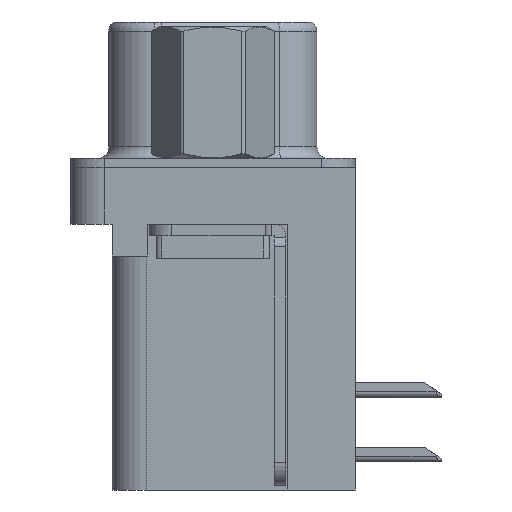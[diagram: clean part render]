
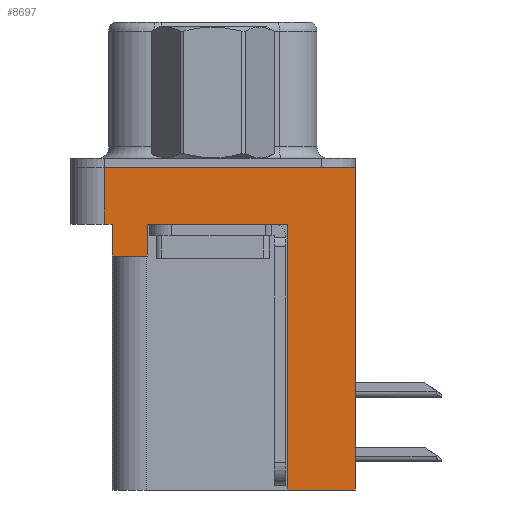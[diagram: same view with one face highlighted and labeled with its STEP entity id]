
A CAD part, left-side view. The second image highlights one B-rep face of the part: STEP entity #8697.
In plain terms, the highlighted planar face has unit normal (-1, 0, 0).
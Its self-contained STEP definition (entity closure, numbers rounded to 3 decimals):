
#73 = DIRECTION ( 'NONE',  ( 0., -1., 0. ) ) ;
#438 = VERTEX_POINT ( 'NONE', #10556 ) ;
#907 = EDGE_LOOP ( 'NONE', ( #11943, #14085, #15891, #15532, #23313, #14474, #13077, #6168, #18651, #9984 ) ) ;
#1224 = EDGE_CURVE ( 'NONE', #3925, #14186, #23632, .T. ) ;
#1886 = CARTESIAN_POINT ( 'NONE',  ( -2.935, -6.275, -2.5 ) ) ;
#2284 = CARTESIAN_POINT ( 'NONE',  ( -2.935, -6.275, 0. ) ) ;
#2301 = CARTESIAN_POINT ( 'NONE',  ( -2.935, -3.295, -14.2 ) ) ;
#2334 = PLANE ( 'NONE',  #7352 ) ;
#2431 = DIRECTION ( 'NONE',  ( 0., -1., 0. ) ) ;
#3066 = VERTEX_POINT ( 'NONE', #3614 ) ;
#3137 = EDGE_CURVE ( 'NONE', #3999, #21410, #13602, .T. ) ;
#3614 = CARTESIAN_POINT ( 'NONE',  ( -2.935, -3.295, -2.5 ) ) ;
#3846 = VECTOR ( 'NONE', #5718, 1000. ) ;
#3925 = VERTEX_POINT ( 'NONE', #4031 ) ;
#3999 = VERTEX_POINT ( 'NONE', #4621 ) ;
#4031 = CARTESIAN_POINT ( 'NONE',  ( -2.935, 4.775, -2.5 ) ) ;
#4054 = LINE ( 'NONE', #18849, #13269 ) ;
#4245 = CARTESIAN_POINT ( 'NONE',  ( -2.935, -6.275, -2.5 ) ) ;
#4557 = VECTOR ( 'NONE', #19603, 1000. ) ;
#4621 = CARTESIAN_POINT ( 'NONE',  ( -2.935, 2.895, -3.9 ) ) ;
#4792 = DIRECTION ( 'NONE',  ( 0., 0., 1. ) ) ;
#5610 = EDGE_CURVE ( 'NONE', #3999, #438, #23203, .T. ) ;
#5718 = DIRECTION ( 'NONE',  ( 0., 0., 1. ) ) ;
#5850 = DIRECTION ( 'NONE',  ( 0., 0., 1. ) ) ;
#6168 = ORIENTED_EDGE ( 'NONE', *, *, #19199, .F. ) ;
#7070 = CARTESIAN_POINT ( 'NONE',  ( -2.935, 2.895, -3.9 ) ) ;
#7352 = AXIS2_PLACEMENT_3D ( 'NONE', #17005, #11230, #18453 ) ;
#7708 = LINE ( 'NONE', #18665, #18121 ) ;
#7763 = VECTOR ( 'NONE', #10112, 1000. ) ;
#8419 = CARTESIAN_POINT ( 'NONE',  ( -2.935, -3.295, -14.2 ) ) ;
#8697 = ADVANCED_FACE ( 'NONE', ( #11104 ), #2334, .T. ) ;
#9215 = CARTESIAN_POINT ( 'NONE',  ( -2.935, 4.425, -3.9 ) ) ;
#9289 = VERTEX_POINT ( 'NONE', #12525 ) ;
#9972 = DIRECTION ( 'NONE',  ( 0., 1., 0. ) ) ;
#9984 = ORIENTED_EDGE ( 'NONE', *, *, #21409, .T. ) ;
#9987 = CARTESIAN_POINT ( 'NONE',  ( -2.935, -3.295, -14.2 ) ) ;
#10095 = VECTOR ( 'NONE', #9972, 1000. ) ;
#10112 = DIRECTION ( 'NONE',  ( 0., 1., 0. ) ) ;
#10114 = LINE ( 'NONE', #9987, #4557 ) ;
#10556 = CARTESIAN_POINT ( 'NONE',  ( -2.935, 2.895, -2.5 ) ) ;
#11104 = FACE_OUTER_BOUND ( 'NONE', #907, .T. ) ;
#11136 = LINE ( 'NONE', #1886, #3846 ) ;
#11230 = DIRECTION ( 'NONE',  ( -1., 0., 0. ) ) ;
#11920 = VECTOR ( 'NONE', #21591, 1000. ) ;
#11943 = ORIENTED_EDGE ( 'NONE', *, *, #23631, .F. ) ;
#12525 = CARTESIAN_POINT ( 'NONE',  ( -2.935, -6.275, -14.2 ) ) ;
#12873 = CARTESIAN_POINT ( 'NONE',  ( -2.935, 4.775, 0. ) ) ;
#13077 = ORIENTED_EDGE ( 'NONE', *, *, #17401, .T. ) ;
#13152 = CARTESIAN_POINT ( 'NONE',  ( -2.935, 4.425, -2.5 ) ) ;
#13269 = VECTOR ( 'NONE', #5850, 1000. ) ;
#13286 = DIRECTION ( 'NONE',  ( 0., -1., 0. ) ) ;
#13307 = EDGE_CURVE ( 'NONE', #21410, #14186, #4054, .T. ) ;
#13602 = LINE ( 'NONE', #19127, #10095 ) ;
#14085 = ORIENTED_EDGE ( 'NONE', *, *, #21740, .F. ) ;
#14131 = CARTESIAN_POINT ( 'NONE',  ( -2.935, 4.775, -2.5 ) ) ;
#14186 = VERTEX_POINT ( 'NONE', #13152 ) ;
#14474 = ORIENTED_EDGE ( 'NONE', *, *, #5610, .T. ) ;
#15532 = ORIENTED_EDGE ( 'NONE', *, *, #13307, .F. ) ;
#15571 = VERTEX_POINT ( 'NONE', #2284 ) ;
#15891 = ORIENTED_EDGE ( 'NONE', *, *, #1224, .T. ) ;
#16053 = VECTOR ( 'NONE', #13286, 1000. ) ;
#16526 = CARTESIAN_POINT ( 'NONE',  ( -2.935, -6.275, -2.5 ) ) ;
#16872 = LINE ( 'NONE', #4245, #16053 ) ;
#16911 = VECTOR ( 'NONE', #73, 1000. ) ;
#17005 = CARTESIAN_POINT ( 'NONE',  ( -2.935, -6.275, -2.5 ) ) ;
#17401 = EDGE_CURVE ( 'NONE', #438, #3066, #16872, .T. ) ;
#18121 = VECTOR ( 'NONE', #2431, 1000. ) ;
#18453 = DIRECTION ( 'NONE',  ( 0., 0., 1. ) ) ;
#18651 = ORIENTED_EDGE ( 'NONE', *, *, #23746, .F. ) ;
#18665 = CARTESIAN_POINT ( 'NONE',  ( -2.935, -6.275, 0. ) ) ;
#18849 = CARTESIAN_POINT ( 'NONE',  ( -2.935, 4.425, -3.9 ) ) ;
#19127 = CARTESIAN_POINT ( 'NONE',  ( -2.935, 4.425, -3.9 ) ) ;
#19199 = EDGE_CURVE ( 'NONE', #23633, #3066, #10114, .T. ) ;
#19603 = DIRECTION ( 'NONE',  ( 0., 0., 1. ) ) ;
#20715 = VECTOR ( 'NONE', #4792, 1000. ) ;
#20780 = VERTEX_POINT ( 'NONE', #12873 ) ;
#21409 = EDGE_CURVE ( 'NONE', #9289, #15571, #11136, .T. ) ;
#21410 = VERTEX_POINT ( 'NONE', #9215 ) ;
#21591 = DIRECTION ( 'NONE',  ( 0., 0., 1. ) ) ;
#21740 = EDGE_CURVE ( 'NONE', #3925, #20780, #22926, .T. ) ;
#22751 = LINE ( 'NONE', #8419, #7763 ) ;
#22926 = LINE ( 'NONE', #14131, #11920 ) ;
#23203 = LINE ( 'NONE', #7070, #20715 ) ;
#23313 = ORIENTED_EDGE ( 'NONE', *, *, #3137, .F. ) ;
#23631 = EDGE_CURVE ( 'NONE', #20780, #15571, #7708, .T. ) ;
#23632 = LINE ( 'NONE', #16526, #16911 ) ;
#23633 = VERTEX_POINT ( 'NONE', #2301 ) ;
#23746 = EDGE_CURVE ( 'NONE', #9289, #23633, #22751, .T. ) ;
